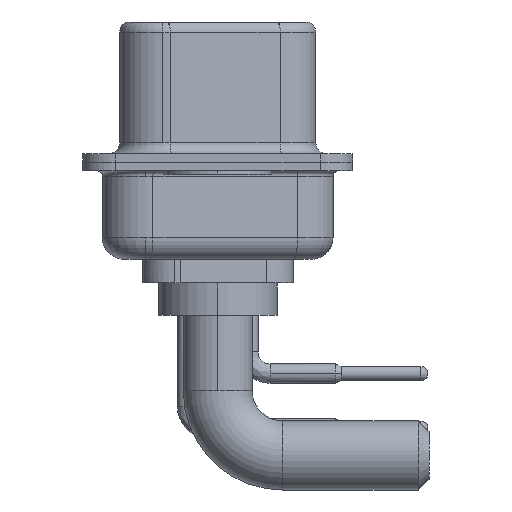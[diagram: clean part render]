
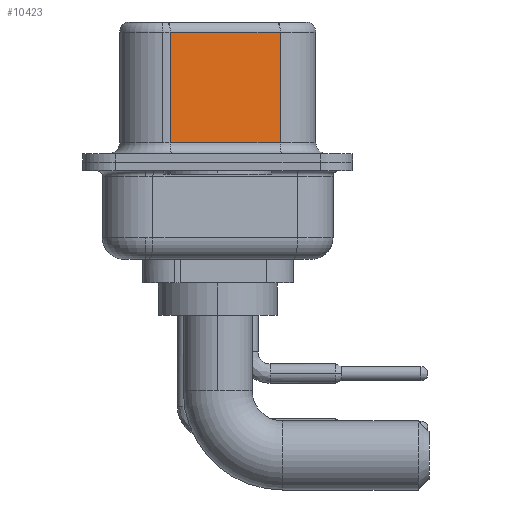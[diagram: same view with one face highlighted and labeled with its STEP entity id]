
A CAD part, left-side view. The second image highlights one B-rep face of the part: STEP entity #10423.
In plain terms, the highlighted planar face has unit normal (-0.985, -0.174, 0).
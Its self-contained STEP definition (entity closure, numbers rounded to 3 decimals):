
#135 = LINE ( 'NONE', #10575, #1607 ) ;
#330 = LINE ( 'NONE', #8398, #24265 ) ;
#1218 = CARTESIAN_POINT ( 'NONE',  ( 3.68, 2.203, 6.52 ) ) ;
#1607 = VECTOR ( 'NONE', #24310, 1000. ) ;
#1766 = VERTEX_POINT ( 'NONE', #18575 ) ;
#4457 = LINE ( 'NONE', #6704, #8507 ) ;
#4925 = EDGE_LOOP ( 'NONE', ( #16007, #21840, #4938, #21956 ) ) ;
#4938 = ORIENTED_EDGE ( 'NONE', *, *, #22618, .T. ) ;
#5546 = EDGE_CURVE ( 'NONE', #13918, #14015, #135, .T. ) ;
#6371 = EDGE_CURVE ( 'NONE', #23863, #1766, #330, .T. ) ;
#6400 = DIRECTION ( 'NONE',  ( -0.174, 0.985, 0. ) ) ;
#6704 = CARTESIAN_POINT ( 'NONE',  ( 4.58, -2.897, 6.52 ) ) ;
#8398 = CARTESIAN_POINT ( 'NONE',  ( 4.58, -2.897, 6.02 ) ) ;
#8507 = VECTOR ( 'NONE', #10680, 1000. ) ;
#8933 = AXIS2_PLACEMENT_3D ( 'NONE', #15887, #26053, #23930 ) ;
#10423 = ADVANCED_FACE ( 'NONE', ( #12043 ), #14159, .F. ) ;
#10575 = CARTESIAN_POINT ( 'NONE',  ( 4.58, -2.897, 0.9 ) ) ;
#10680 = DIRECTION ( 'NONE',  ( 0., 0., -1. ) ) ;
#12043 = FACE_OUTER_BOUND ( 'NONE', #4925, .T. ) ;
#13440 = CARTESIAN_POINT ( 'NONE',  ( 4.58, -2.897, 0.9 ) ) ;
#13918 = VERTEX_POINT ( 'NONE', #23329 ) ;
#14015 = VERTEX_POINT ( 'NONE', #13440 ) ;
#14159 = PLANE ( 'NONE',  #8933 ) ;
#15384 = LINE ( 'NONE', #1218, #25876 ) ;
#15887 = CARTESIAN_POINT ( 'NONE',  ( 4.58, -2.897, 6.52 ) ) ;
#16007 = ORIENTED_EDGE ( 'NONE', *, *, #21504, .F. ) ;
#17322 = CARTESIAN_POINT ( 'NONE',  ( 4.58, -2.897, 6.02 ) ) ;
#18575 = CARTESIAN_POINT ( 'NONE',  ( 3.68, 2.203, 6.02 ) ) ;
#21437 = DIRECTION ( 'NONE',  ( 0., 0., -1. ) ) ;
#21504 = EDGE_CURVE ( 'NONE', #23863, #14015, #4457, .T. ) ;
#21840 = ORIENTED_EDGE ( 'NONE', *, *, #6371, .T. ) ;
#21956 = ORIENTED_EDGE ( 'NONE', *, *, #5546, .T. ) ;
#22618 = EDGE_CURVE ( 'NONE', #1766, #13918, #15384, .T. ) ;
#23329 = CARTESIAN_POINT ( 'NONE',  ( 3.68, 2.203, 0.9 ) ) ;
#23863 = VERTEX_POINT ( 'NONE', #17322 ) ;
#23930 = DIRECTION ( 'NONE',  ( -0.174, 0.985, 0. ) ) ;
#24265 = VECTOR ( 'NONE', #6400, 1000. ) ;
#24310 = DIRECTION ( 'NONE',  ( 0.174, -0.985, 0. ) ) ;
#25876 = VECTOR ( 'NONE', #21437, 1000. ) ;
#26053 = DIRECTION ( 'NONE',  ( 0.985, 0.174, 0. ) ) ;
